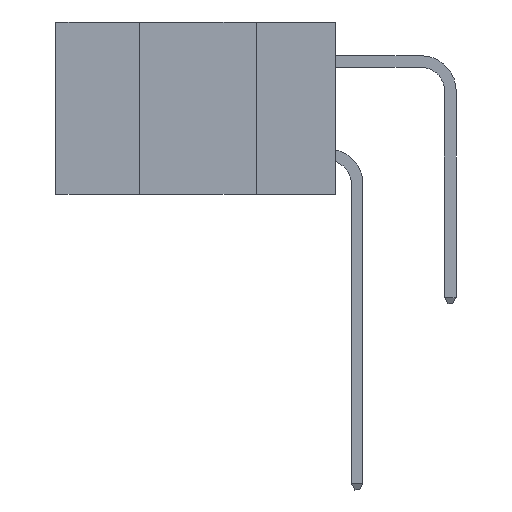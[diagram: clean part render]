
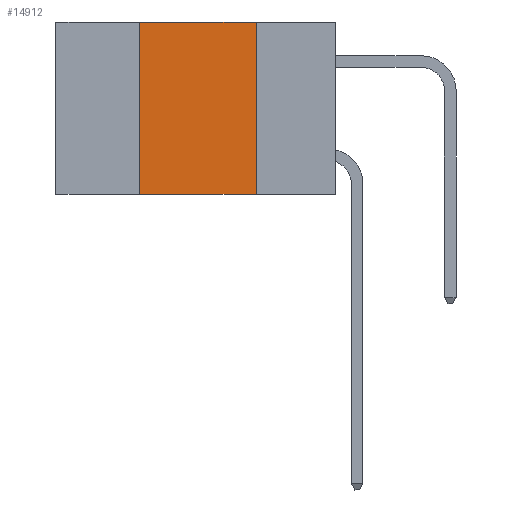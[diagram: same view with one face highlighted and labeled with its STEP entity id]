
A CAD part, left-side view. The second image highlights one B-rep face of the part: STEP entity #14912.
In plain terms, the highlighted planar face has unit normal (-1, 0, 0).
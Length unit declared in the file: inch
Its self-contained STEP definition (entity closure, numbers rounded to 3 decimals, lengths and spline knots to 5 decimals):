
#821 = ORIENTED_EDGE ( 'NONE', *, *, #5823, .F. ) ;
#1005 = DIRECTION ( 'NONE',  ( 1., 0., 0. ) ) ;
#1699 = LINE ( 'NONE', #14869, #10175 ) ;
#2391 = LINE ( 'NONE', #10964, #4581 ) ;
#4581 = VECTOR ( 'NONE', #9854, 39.37008 ) ;
#5173 = EDGE_LOOP ( 'NONE', ( #821, #13588, #9250, #12760 ) ) ;
#5470 = EDGE_CURVE ( 'NONE', #15565, #7839, #15210, .T. ) ;
#5823 = EDGE_CURVE ( 'NONE', #7839, #14911, #1699, .T. ) ;
#6076 = EDGE_CURVE ( 'NONE', #12150, #14911, #2391, .T. ) ;
#7163 = DIRECTION ( 'NONE',  ( 0., 0., 1. ) ) ;
#7839 = VERTEX_POINT ( 'NONE', #8643 ) ;
#8069 = DIRECTION ( 'NONE',  ( 0., -1., 0. ) ) ;
#8517 = LINE ( 'NONE', #13353, #10094 ) ;
#8643 = CARTESIAN_POINT ( 'NONE',  ( 0., 0.17, 0. ) ) ;
#8721 = AXIS2_PLACEMENT_3D ( 'NONE', #15446, #1005, #9340 ) ;
#9250 = ORIENTED_EDGE ( 'NONE', *, *, #11744, .F. ) ;
#9340 = DIRECTION ( 'NONE',  ( 0., 0., -1. ) ) ;
#9854 = DIRECTION ( 'NONE',  ( 0., -1., 0. ) ) ;
#10094 = VECTOR ( 'NONE', #7163, 39.37008 ) ;
#10175 = VECTOR ( 'NONE', #11142, 39.37008 ) ;
#10964 = CARTESIAN_POINT ( 'NONE',  ( 0., 0.6, -0.37 ) ) ;
#11142 = DIRECTION ( 'NONE',  ( 0., 0., -1. ) ) ;
#11744 = EDGE_CURVE ( 'NONE', #12150, #15565, #8517, .T. ) ;
#11879 = FACE_OUTER_BOUND ( 'NONE', #5173, .T. ) ;
#11993 = CARTESIAN_POINT ( 'NONE',  ( 0., 0.42, -0.37 ) ) ;
#12150 = VERTEX_POINT ( 'NONE', #11993 ) ;
#12760 = ORIENTED_EDGE ( 'NONE', *, *, #6076, .T. ) ;
#12761 = CARTESIAN_POINT ( 'NONE',  ( 0., 0.42, 0. ) ) ;
#12906 = CARTESIAN_POINT ( 'NONE',  ( 0., 0.17, -0.37 ) ) ;
#13353 = CARTESIAN_POINT ( 'NONE',  ( 0., 0.42, 0. ) ) ;
#13588 = ORIENTED_EDGE ( 'NONE', *, *, #5470, .F. ) ;
#14010 = PLANE ( 'NONE',  #8721 ) ;
#14012 = CARTESIAN_POINT ( 'NONE',  ( 0., 0.6, 0. ) ) ;
#14869 = CARTESIAN_POINT ( 'NONE',  ( 0., 0.17, 0. ) ) ;
#14911 = VERTEX_POINT ( 'NONE', #12906 ) ;
#14912 = ADVANCED_FACE ( 'NONE', ( #11879 ), #14010, .F. ) ;
#15210 = LINE ( 'NONE', #14012, #15258 ) ;
#15258 = VECTOR ( 'NONE', #8069, 39.37008 ) ;
#15446 = CARTESIAN_POINT ( 'NONE',  ( 0., 0.6, 0. ) ) ;
#15565 = VERTEX_POINT ( 'NONE', #12761 ) ;
